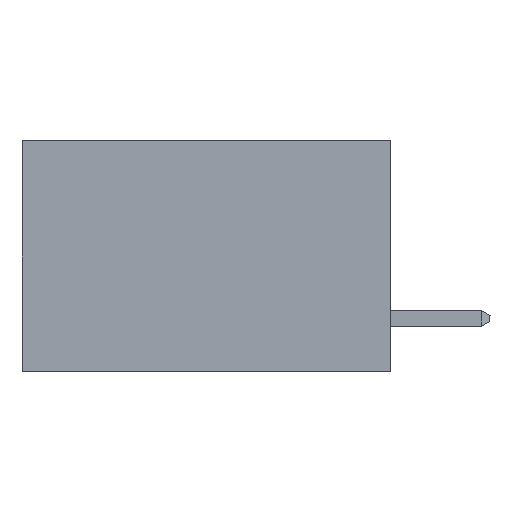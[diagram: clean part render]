
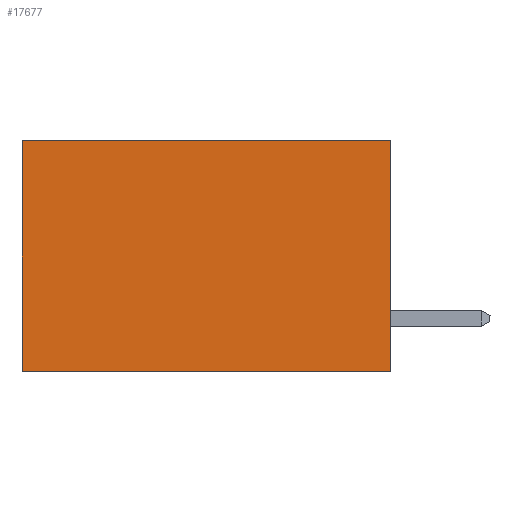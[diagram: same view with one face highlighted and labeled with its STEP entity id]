
A CAD part, left-side view. The second image highlights one B-rep face of the part: STEP entity #17677.
In plain terms, the highlighted planar face has unit normal (-1, 0, 0).
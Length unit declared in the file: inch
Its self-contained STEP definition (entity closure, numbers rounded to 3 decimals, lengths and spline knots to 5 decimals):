
#352 = VECTOR ( 'NONE', #6651, 39.37008 ) ;
#928 = CARTESIAN_POINT ( 'NONE',  ( 0.277, 0.59, -0.37 ) ) ;
#1638 = DIRECTION ( 'NONE',  ( 0., 0., -1. ) ) ;
#1689 = CARTESIAN_POINT ( 'NONE',  ( 0.277, 0., -0.37 ) ) ;
#3136 = DIRECTION ( 'NONE',  ( 0., 1., 0. ) ) ;
#4567 = VECTOR ( 'NONE', #3136, 39.37008 ) ;
#4595 = FACE_OUTER_BOUND ( 'NONE', #23077, .T. ) ;
#5075 = CARTESIAN_POINT ( 'NONE',  ( 0.277, 0.59, -0.37 ) ) ;
#6311 = VERTEX_POINT ( 'NONE', #25608 ) ;
#6651 = DIRECTION ( 'NONE',  ( 0., 0., -1. ) ) ;
#7549 = LINE ( 'NONE', #5075, #11200 ) ;
#9419 = CARTESIAN_POINT ( 'NONE',  ( 0.277, 0., 0. ) ) ;
#11200 = VECTOR ( 'NONE', #22225, 39.37008 ) ;
#12271 = ORIENTED_EDGE ( 'NONE', *, *, #15277, .F. ) ;
#12386 = LINE ( 'NONE', #23784, #352 ) ;
#12824 = AXIS2_PLACEMENT_3D ( 'NONE', #27234, #14450, #1638 ) ;
#14450 = DIRECTION ( 'NONE',  ( 1., 0., 0. ) ) ;
#15277 = EDGE_CURVE ( 'NONE', #24840, #21831, #12386, .T. ) ;
#16409 = CARTESIAN_POINT ( 'NONE',  ( 0.277, 0., -0.37 ) ) ;
#16851 = CARTESIAN_POINT ( 'NONE',  ( 0.277, 0., 0. ) ) ;
#17677 = ADVANCED_FACE ( 'NONE', ( #4595 ), #22990, .F. ) ;
#18152 = EDGE_CURVE ( 'NONE', #24840, #6311, #21005, .T. ) ;
#18555 = DIRECTION ( 'NONE',  ( 0., 1., 0. ) ) ;
#19563 = ORIENTED_EDGE ( 'NONE', *, *, #24508, .T. ) ;
#19835 = VECTOR ( 'NONE', #18555, 39.37008 ) ;
#21005 = LINE ( 'NONE', #9419, #4567 ) ;
#21831 = VERTEX_POINT ( 'NONE', #1689 ) ;
#22090 = ORIENTED_EDGE ( 'NONE', *, *, #18152, .T. ) ;
#22225 = DIRECTION ( 'NONE',  ( 0., 0., -1. ) ) ;
#22284 = ORIENTED_EDGE ( 'NONE', *, *, #26968, .F. ) ;
#22990 = PLANE ( 'NONE',  #12824 ) ;
#23077 = EDGE_LOOP ( 'NONE', ( #19563, #22284, #12271, #22090 ) ) ;
#23784 = CARTESIAN_POINT ( 'NONE',  ( 0.277, 0., -0.37 ) ) ;
#24508 = EDGE_CURVE ( 'NONE', #6311, #27490, #7549, .T. ) ;
#24840 = VERTEX_POINT ( 'NONE', #16851 ) ;
#25608 = CARTESIAN_POINT ( 'NONE',  ( 0.277, 0.59, 0. ) ) ;
#26175 = LINE ( 'NONE', #16409, #19835 ) ;
#26968 = EDGE_CURVE ( 'NONE', #21831, #27490, #26175, .T. ) ;
#27234 = CARTESIAN_POINT ( 'NONE',  ( 0.277, 0., -0.37 ) ) ;
#27490 = VERTEX_POINT ( 'NONE', #928 ) ;
